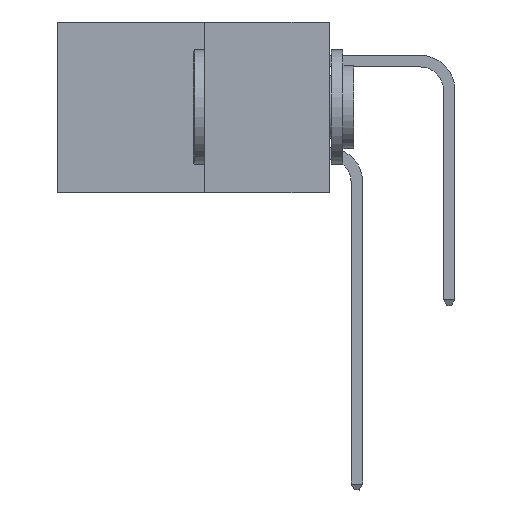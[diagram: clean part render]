
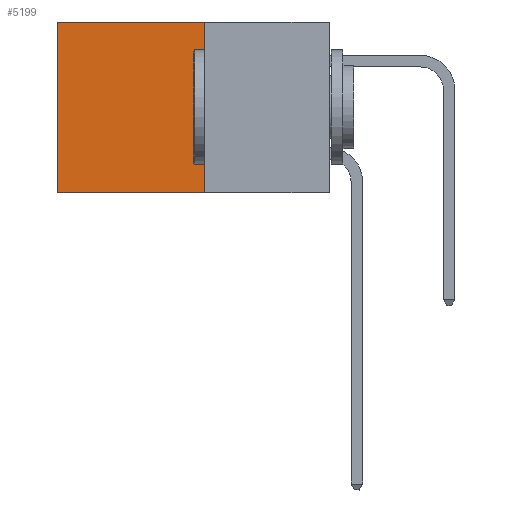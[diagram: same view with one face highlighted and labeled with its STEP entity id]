
A CAD part, left-side view. The second image highlights one B-rep face of the part: STEP entity #5199.
In plain terms, the highlighted planar face has unit normal (-1, 0, 0).
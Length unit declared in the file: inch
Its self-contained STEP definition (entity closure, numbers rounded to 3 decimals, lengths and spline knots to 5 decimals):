
#955 = LINE ( 'NONE', #6602, #16306 ) ;
#1174 = VERTEX_POINT ( 'NONE', #1756 ) ;
#1756 = CARTESIAN_POINT ( 'NONE',  ( 0.277, 0.59, -0.37 ) ) ;
#3144 = EDGE_CURVE ( 'NONE', #8797, #1174, #12942, .T. ) ;
#3381 = CARTESIAN_POINT ( 'NONE',  ( 0.277, 0.27, 0. ) ) ;
#3945 = LINE ( 'NONE', #5834, #11373 ) ;
#4033 = VERTEX_POINT ( 'NONE', #3381 ) ;
#4830 = PLANE ( 'NONE',  #7583 ) ;
#5199 = ADVANCED_FACE ( 'NONE', ( #6726 ), #4830, .F. ) ;
#5585 = EDGE_LOOP ( 'NONE', ( #11379, #13034, #7556, #9818 ) ) ;
#5834 = CARTESIAN_POINT ( 'NONE',  ( 0.277, 0.27, -0.37 ) ) ;
#6170 = CARTESIAN_POINT ( 'NONE',  ( 0.277, 0.27, -0.37 ) ) ;
#6602 = CARTESIAN_POINT ( 'NONE',  ( 0.277, 0.27, 0. ) ) ;
#6726 = FACE_OUTER_BOUND ( 'NONE', #5585, .T. ) ;
#6923 = CARTESIAN_POINT ( 'NONE',  ( 0.277, 0.27, -0.37 ) ) ;
#7556 = ORIENTED_EDGE ( 'NONE', *, *, #11115, .F. ) ;
#7583 = AXIS2_PLACEMENT_3D ( 'NONE', #15121, #16627, #7858 ) ;
#7858 = DIRECTION ( 'NONE',  ( 0., 0., -1. ) ) ;
#8718 = CARTESIAN_POINT ( 'NONE',  ( 0.277, 0.59, 0. ) ) ;
#8797 = VERTEX_POINT ( 'NONE', #6923 ) ;
#8816 = CARTESIAN_POINT ( 'NONE',  ( 0.277, 0.59, -0.37 ) ) ;
#9818 = ORIENTED_EDGE ( 'NONE', *, *, #15117, .T. ) ;
#10248 = DIRECTION ( 'NONE',  ( 0., 0., -1. ) ) ;
#10316 = DIRECTION ( 'NONE',  ( 0., 0., -1. ) ) ;
#11115 = EDGE_CURVE ( 'NONE', #4033, #8797, #3945, .T. ) ;
#11373 = VECTOR ( 'NONE', #10316, 39.37008 ) ;
#11379 = ORIENTED_EDGE ( 'NONE', *, *, #13126, .T. ) ;
#11508 = LINE ( 'NONE', #8816, #14937 ) ;
#11621 = DIRECTION ( 'NONE',  ( 0., 1., 0. ) ) ;
#12942 = LINE ( 'NONE', #6170, #16414 ) ;
#13034 = ORIENTED_EDGE ( 'NONE', *, *, #3144, .F. ) ;
#13126 = EDGE_CURVE ( 'NONE', #16774, #1174, #11508, .T. ) ;
#14937 = VECTOR ( 'NONE', #10248, 39.37008 ) ;
#15117 = EDGE_CURVE ( 'NONE', #4033, #16774, #955, .T. ) ;
#15121 = CARTESIAN_POINT ( 'NONE',  ( 0.277, 0.27, -0.37 ) ) ;
#15418 = DIRECTION ( 'NONE',  ( 0., 1., 0. ) ) ;
#16306 = VECTOR ( 'NONE', #15418, 39.37008 ) ;
#16414 = VECTOR ( 'NONE', #11621, 39.37008 ) ;
#16627 = DIRECTION ( 'NONE',  ( 1., 0., 0. ) ) ;
#16774 = VERTEX_POINT ( 'NONE', #8718 ) ;
